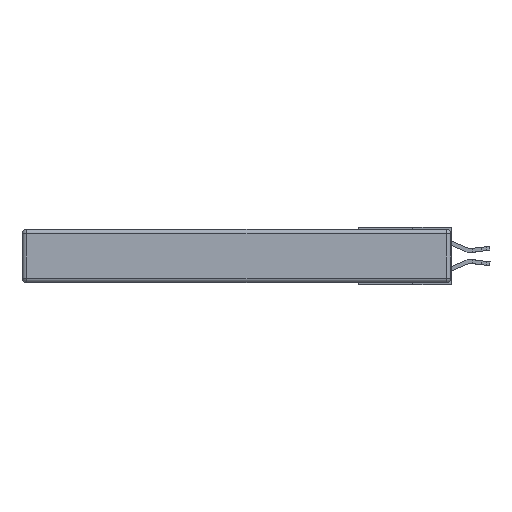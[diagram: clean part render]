
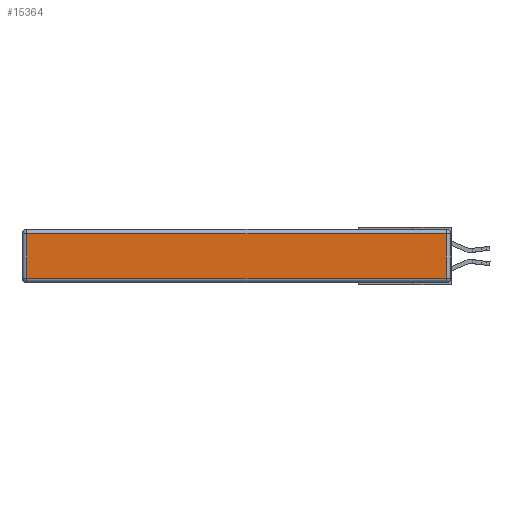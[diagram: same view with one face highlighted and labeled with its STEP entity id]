
A CAD part, left-side view. The second image highlights one B-rep face of the part: STEP entity #15364.
In plain terms, the highlighted planar face has unit normal (-1, 0, 0).
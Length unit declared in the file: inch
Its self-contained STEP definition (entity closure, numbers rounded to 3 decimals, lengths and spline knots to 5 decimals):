
#421 = DIRECTION ( 'NONE',  ( 0., 1., 0. ) ) ;
#509 = EDGE_CURVE ( 'NONE', #13551, #1955, #1785, .T. ) ;
#1234 = CARTESIAN_POINT ( 'NONE',  ( 0., 2.72, -0.03 ) ) ;
#1570 = ORIENTED_EDGE ( 'NONE', *, *, #3596, .T. ) ;
#1785 = LINE ( 'NONE', #11081, #14372 ) ;
#1921 = DIRECTION ( 'NONE',  ( -1., 0., 0. ) ) ;
#1955 = VERTEX_POINT ( 'NONE', #10315 ) ;
#2945 = CARTESIAN_POINT ( 'NONE',  ( 0., 0., -0.313 ) ) ;
#3514 = FACE_OUTER_BOUND ( 'NONE', #16165, .T. ) ;
#3596 = EDGE_CURVE ( 'NONE', #9208, #13551, #14915, .T. ) ;
#3628 = LINE ( 'NONE', #2945, #4256 ) ;
#3874 = DIRECTION ( 'NONE',  ( 0., 0., -1. ) ) ;
#3885 = EDGE_CURVE ( 'NONE', #1955, #17012, #3628, .T. ) ;
#4256 = VECTOR ( 'NONE', #17064, 39.37008 ) ;
#4804 = CARTESIAN_POINT ( 'NONE',  ( 0., 0., -0.343 ) ) ;
#5562 = DIRECTION ( 'NONE',  ( 0., 0., 1. ) ) ;
#7122 = CARTESIAN_POINT ( 'NONE',  ( 0., 0.03, -0.343 ) ) ;
#7287 = ORIENTED_EDGE ( 'NONE', *, *, #509, .T. ) ;
#7443 = ORIENTED_EDGE ( 'NONE', *, *, #7875, .T. ) ;
#7875 = EDGE_CURVE ( 'NONE', #17012, #9208, #10072, .T. ) ;
#8992 = PLANE ( 'NONE',  #15149 ) ;
#9208 = VERTEX_POINT ( 'NONE', #13352 ) ;
#10072 = LINE ( 'NONE', #7122, #11402 ) ;
#10315 = CARTESIAN_POINT ( 'NONE',  ( 0., 2.72, -0.313 ) ) ;
#11047 = ORIENTED_EDGE ( 'NONE', *, *, #3885, .T. ) ;
#11081 = CARTESIAN_POINT ( 'NONE',  ( 0., 2.72, -0.343 ) ) ;
#11402 = VECTOR ( 'NONE', #5562, 39.37008 ) ;
#11819 = CARTESIAN_POINT ( 'NONE',  ( 0., 0.03, -0.313 ) ) ;
#13352 = CARTESIAN_POINT ( 'NONE',  ( 0., 0.03, -0.03 ) ) ;
#13551 = VERTEX_POINT ( 'NONE', #1234 ) ;
#14025 = VECTOR ( 'NONE', #421, 39.37008 ) ;
#14372 = VECTOR ( 'NONE', #3874, 39.37008 ) ;
#14915 = LINE ( 'NONE', #16900, #14025 ) ;
#15149 = AXIS2_PLACEMENT_3D ( 'NONE', #4804, #1921, #17314 ) ;
#15364 = ADVANCED_FACE ( 'NONE', ( #3514 ), #8992, .T. ) ;
#16165 = EDGE_LOOP ( 'NONE', ( #11047, #7443, #1570, #7287 ) ) ;
#16900 = CARTESIAN_POINT ( 'NONE',  ( 0., 2.75, -0.03 ) ) ;
#17012 = VERTEX_POINT ( 'NONE', #11819 ) ;
#17064 = DIRECTION ( 'NONE',  ( 0., -1., 0. ) ) ;
#17314 = DIRECTION ( 'NONE',  ( 0., 0., 1. ) ) ;
